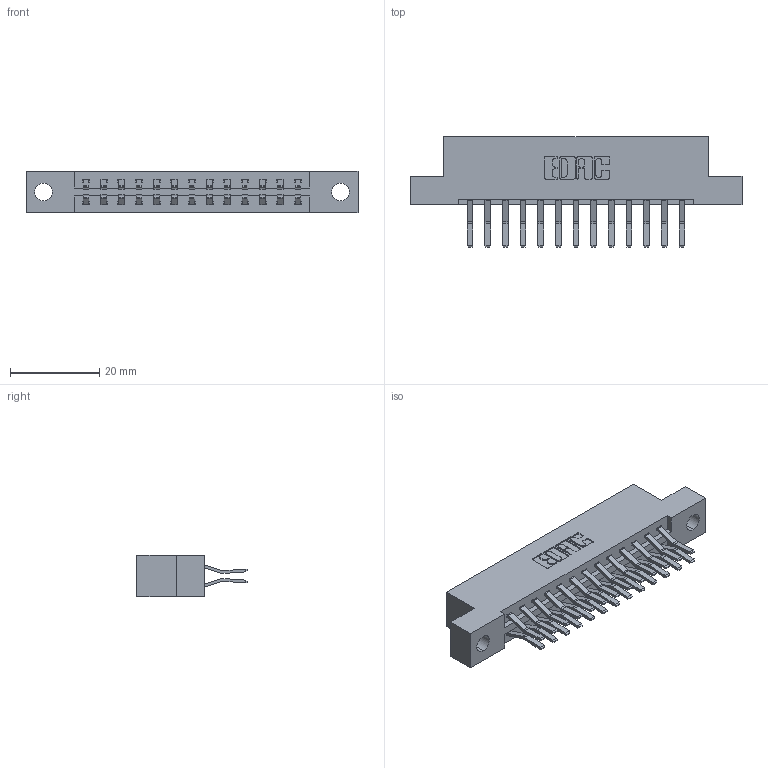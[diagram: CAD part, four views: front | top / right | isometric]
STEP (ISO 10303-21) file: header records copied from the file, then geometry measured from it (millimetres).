
FILE_DESCRIPTION (( 'STEP AP203' ), '1' );
FILE_NAME ('387-026-560-204.STEP', '2018-09-16T13:00:42', ( '' ), ( '' ), 'SwSTEP 2.0', 'SolidWorks 2016', '' );
FILE_SCHEMA (( 'CONFIG_CONTROL_DESIGN' ));
Length unit declared in the file: inch
Products named in the file (3): 387-026-560-204; 337 Part_Flush Mounting Lugs - 0.156 Dia-TH; 345-292-001_560 Tail
Assembly tree (27 placements, depth 2):
  387-026-560-204
    337 Part_Flush Mounting Lugs - 0.156 Dia-TH
    345-292-001_560 Tail  x26
Bounding box: 74.52 x 24.78 x 9.4 mm (x, y, z)
Volume: 7550.4 mm3; surface area: 8544.7 mm2
Topology: 27 solids, 27 shells, 1570 faces, 4653 edges, 3066 vertices
Faces by surface type: plane 1058, cylinder 512
Entity records: 13921 total; most frequent: CARTESIAN_POINT 2370, ORIENTED_EDGE 2306, DIRECTION 2073, EDGE_CURVE 1153, VECTOR 1021, LINE 1021, VERTEX_POINT 766, AXIS2_PLACEMENT_3D 526
